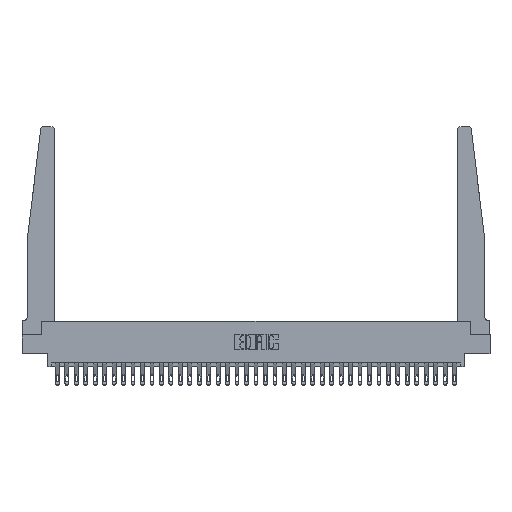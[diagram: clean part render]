
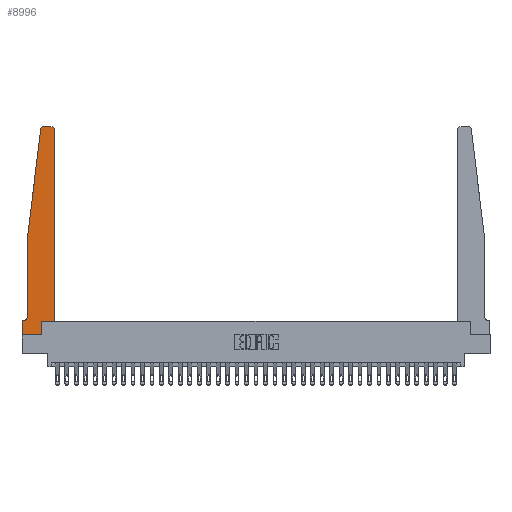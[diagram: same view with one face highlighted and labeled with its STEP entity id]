
A CAD part, top view. The second image highlights one B-rep face of the part: STEP entity #8996.
In plain terms, the highlighted planar face has unit normal (0, 0, 1).
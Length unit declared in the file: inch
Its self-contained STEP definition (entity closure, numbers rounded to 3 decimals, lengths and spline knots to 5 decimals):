
#636 = CARTESIAN_POINT ( 'NONE',  ( 0.015, 0.2375, 0.37 ) ) ;
#757 = ORIENTED_EDGE ( 'NONE', *, *, #21042, .T. ) ;
#777 = EDGE_CURVE ( 'NONE', #17055, #19957, #9194, .T. ) ;
#1000 = CARTESIAN_POINT ( 'NONE',  ( 0.2605, 0.18, 0.37 ) ) ;
#2066 = LINE ( 'NONE', #2558, #25480 ) ;
#2558 = CARTESIAN_POINT ( 'NONE',  ( 0., 0., 0.37 ) ) ;
#3269 = LINE ( 'NONE', #29146, #13132 ) ;
#3336 = DIRECTION ( 'NONE',  ( 1., 0., 0. ) ) ;
#3573 = CARTESIAN_POINT ( 'NONE',  ( 0.065, 0.2375, 0.37 ) ) ;
#3654 = AXIS2_PLACEMENT_3D ( 'NONE', #27338, #14380, #3336 ) ;
#4274 = ORIENTED_EDGE ( 'NONE', *, *, #24103, .T. ) ;
#4373 = DIRECTION ( 'NONE',  ( -1., 0., 0. ) ) ;
#4466 = CARTESIAN_POINT ( 'NONE',  ( 0.27653, 2.72, 0.37 ) ) ;
#4523 = VECTOR ( 'NONE', #14283, 39.37008 ) ;
#4670 = VECTOR ( 'NONE', #4373, 39.37008 ) ;
#5243 = VERTEX_POINT ( 'NONE', #6991 ) ;
#5743 = ORIENTED_EDGE ( 'NONE', *, *, #18890, .T. ) ;
#5784 = LINE ( 'NONE', #7827, #17205 ) ;
#6474 = AXIS2_PLACEMENT_3D ( 'NONE', #4466, #11937, #14824 ) ;
#6554 = FACE_OUTER_BOUND ( 'NONE', #13179, .T. ) ;
#6991 = CARTESIAN_POINT ( 'NONE',  ( 0.065, 1.25, 0.37 ) ) ;
#7215 = DIRECTION ( 'NONE',  ( 0., 0., 1. ) ) ;
#7778 = DIRECTION ( 'NONE',  ( 0., 0., -1. ) ) ;
#7827 = CARTESIAN_POINT ( 'NONE',  ( 0., 0., 0.37 ) ) ;
#7924 = CARTESIAN_POINT ( 'NONE',  ( 0.2605, 0.18, 0.37 ) ) ;
#7947 = DIRECTION ( 'NONE',  ( -1., 0., 0. ) ) ;
#8526 = CIRCLE ( 'NONE', #21018, 0.03 ) ;
#8814 = VECTOR ( 'NONE', #21209, 39.37008 ) ;
#8963 = DIRECTION ( 'NONE',  ( 0., -1., 0. ) ) ;
#8996 = ADVANCED_FACE ( 'NONE', ( #6554 ), #16928, .T. ) ;
#9194 = CIRCLE ( 'NONE', #6474, 0.03 ) ;
#9417 = VERTEX_POINT ( 'NONE', #17623 ) ;
#10239 = EDGE_CURVE ( 'NONE', #20101, #30232, #14780, .T. ) ;
#10772 = ORIENTED_EDGE ( 'NONE', *, *, #33197, .T. ) ;
#11028 = AXIS2_PLACEMENT_3D ( 'NONE', #636, #7778, #7947 ) ;
#11124 = VECTOR ( 'NONE', #8963, 39.37008 ) ;
#11345 = CARTESIAN_POINT ( 'NONE',  ( 0.065, 1.25, 0.37 ) ) ;
#11937 = DIRECTION ( 'NONE',  ( 0., 0., 1. ) ) ;
#12666 = CARTESIAN_POINT ( 'NONE',  ( 0.395, 2.72, 0.37 ) ) ;
#13000 = DIRECTION ( 'NONE',  ( 1., 0., 0. ) ) ;
#13132 = VECTOR ( 'NONE', #21139, 39.37008 ) ;
#13179 = EDGE_LOOP ( 'NONE', ( #17282, #33208, #4274, #10772, #26084, #30541, #15648, #757, #32307, #20634, #30349, #5743 ) ) ;
#13557 = CARTESIAN_POINT ( 'NONE',  ( 0.25, 2.75, 0.37 ) ) ;
#13919 = VECTOR ( 'NONE', #31339, 39.37008 ) ;
#14052 = DIRECTION ( 'NONE',  ( -1., 0., 0. ) ) ;
#14283 = DIRECTION ( 'NONE',  ( 1., 0., 0. ) ) ;
#14380 = DIRECTION ( 'NONE',  ( 0., 0., 1. ) ) ;
#14780 = LINE ( 'NONE', #22611, #4523 ) ;
#14824 = DIRECTION ( 'NONE',  ( 1., 0., 0. ) ) ;
#15427 = EDGE_CURVE ( 'NONE', #18897, #27230, #17278, .T. ) ;
#15648 = ORIENTED_EDGE ( 'NONE', *, *, #16585, .T. ) ;
#16585 = EDGE_CURVE ( 'NONE', #27230, #9417, #5784, .T. ) ;
#16685 = CARTESIAN_POINT ( 'NONE',  ( 0.395, 2.75, 0.37 ) ) ;
#16928 = PLANE ( 'NONE',  #3654 ) ;
#17055 = VERTEX_POINT ( 'NONE', #26510 ) ;
#17205 = VECTOR ( 'NONE', #18202, 39.37008 ) ;
#17278 = LINE ( 'NONE', #24965, #4670 ) ;
#17282 = ORIENTED_EDGE ( 'NONE', *, *, #23290, .T. ) ;
#17417 = VECTOR ( 'NONE', #14052, 39.37008 ) ;
#17623 = CARTESIAN_POINT ( 'NONE',  ( 0., 0., 0.37 ) ) ;
#18109 = EDGE_CURVE ( 'NONE', #30232, #30028, #23503, .T. ) ;
#18202 = DIRECTION ( 'NONE',  ( 0., -1., 0. ) ) ;
#18366 = VERTEX_POINT ( 'NONE', #3573 ) ;
#18728 = VERTEX_POINT ( 'NONE', #29716 ) ;
#18890 = EDGE_CURVE ( 'NONE', #30028, #29793, #8526, .T. ) ;
#18897 = VERTEX_POINT ( 'NONE', #33426 ) ;
#19957 = VERTEX_POINT ( 'NONE', #23630 ) ;
#20101 = VERTEX_POINT ( 'NONE', #1000 ) ;
#20634 = ORIENTED_EDGE ( 'NONE', *, *, #10239, .T. ) ;
#21018 = AXIS2_PLACEMENT_3D ( 'NONE', #12666, #7215, #13000 ) ;
#21042 = EDGE_CURVE ( 'NONE', #9417, #18728, #2066, .T. ) ;
#21139 = DIRECTION ( 'NONE',  ( -0.122, -0.992, 0. ) ) ;
#21209 = DIRECTION ( 'NONE',  ( 0., 1., 0. ) ) ;
#22611 = CARTESIAN_POINT ( 'NONE',  ( 0.425, 0.18, 0.37 ) ) ;
#23290 = EDGE_CURVE ( 'NONE', #29793, #17055, #26833, .T. ) ;
#23503 = LINE ( 'NONE', #23663, #13919 ) ;
#23630 = CARTESIAN_POINT ( 'NONE',  ( 0.24675, 2.72367, 0.37 ) ) ;
#23663 = CARTESIAN_POINT ( 'NONE',  ( 0.425, 0.18, 0.37 ) ) ;
#23747 = LINE ( 'NONE', #7924, #8814 ) ;
#24103 = EDGE_CURVE ( 'NONE', #19957, #5243, #3269, .T. ) ;
#24965 = CARTESIAN_POINT ( 'NONE',  ( 0.065, 0.1875, 0.37 ) ) ;
#24974 = LINE ( 'NONE', #11345, #11124 ) ;
#25480 = VECTOR ( 'NONE', #27761, 39.37008 ) ;
#26084 = ORIENTED_EDGE ( 'NONE', *, *, #30590, .T. ) ;
#26294 = CIRCLE ( 'NONE', #11028, 0.05 ) ;
#26510 = CARTESIAN_POINT ( 'NONE',  ( 0.27653, 2.75, 0.37 ) ) ;
#26833 = LINE ( 'NONE', #13557, #17417 ) ;
#26987 = EDGE_CURVE ( 'NONE', #18728, #20101, #23747, .T. ) ;
#27230 = VERTEX_POINT ( 'NONE', #28343 ) ;
#27338 = CARTESIAN_POINT ( 'NONE',  ( 0., 0.1875, 0.37 ) ) ;
#27761 = DIRECTION ( 'NONE',  ( 1., 0., 0. ) ) ;
#28343 = CARTESIAN_POINT ( 'NONE',  ( 0., 0.1875, 0.37 ) ) ;
#29146 = CARTESIAN_POINT ( 'NONE',  ( 0.065, 1.25, 0.37 ) ) ;
#29267 = CARTESIAN_POINT ( 'NONE',  ( 0.425, 2.72, 0.37 ) ) ;
#29716 = CARTESIAN_POINT ( 'NONE',  ( 0.2605, 0., 0.37 ) ) ;
#29793 = VERTEX_POINT ( 'NONE', #16685 ) ;
#30028 = VERTEX_POINT ( 'NONE', #29267 ) ;
#30232 = VERTEX_POINT ( 'NONE', #32656 ) ;
#30349 = ORIENTED_EDGE ( 'NONE', *, *, #18109, .T. ) ;
#30541 = ORIENTED_EDGE ( 'NONE', *, *, #15427, .T. ) ;
#30590 = EDGE_CURVE ( 'NONE', #18366, #18897, #26294, .T. ) ;
#31339 = DIRECTION ( 'NONE',  ( 0., 1., 0. ) ) ;
#32307 = ORIENTED_EDGE ( 'NONE', *, *, #26987, .T. ) ;
#32656 = CARTESIAN_POINT ( 'NONE',  ( 0.425, 0.18, 0.37 ) ) ;
#33197 = EDGE_CURVE ( 'NONE', #5243, #18366, #24974, .T. ) ;
#33208 = ORIENTED_EDGE ( 'NONE', *, *, #777, .T. ) ;
#33426 = CARTESIAN_POINT ( 'NONE',  ( 0.015, 0.1875, 0.37 ) ) ;
